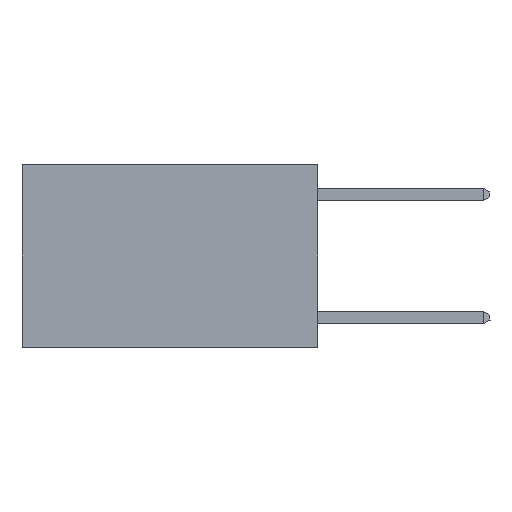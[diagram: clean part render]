
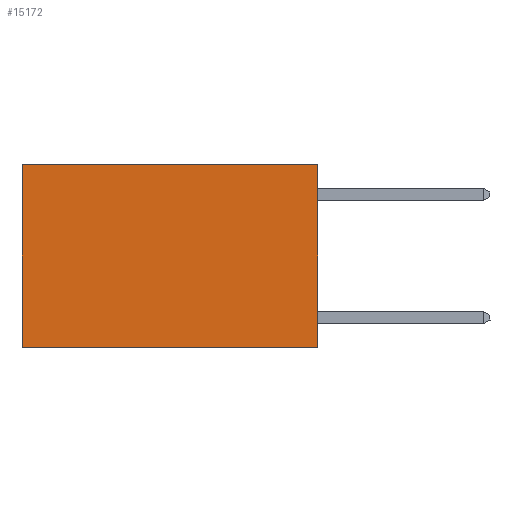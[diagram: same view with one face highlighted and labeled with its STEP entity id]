
A CAD part, left-side view. The second image highlights one B-rep face of the part: STEP entity #15172.
In plain terms, the highlighted planar face has unit normal (-1, 0, 0).
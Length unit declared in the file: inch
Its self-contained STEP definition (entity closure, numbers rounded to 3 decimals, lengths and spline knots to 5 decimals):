
#1443 = DIRECTION ( 'NONE',  ( 0., 1., 0. ) ) ;
#1890 = VECTOR ( 'NONE', #13519, 39.37008 ) ;
#2534 = AXIS2_PLACEMENT_3D ( 'NONE', #2882, #6406, #18572 ) ;
#2811 = PLANE ( 'NONE',  #2534 ) ;
#2882 = CARTESIAN_POINT ( 'NONE',  ( 0.2625, 0., 0. ) ) ;
#3169 = CARTESIAN_POINT ( 'NONE',  ( 0.2625, 0., 0. ) ) ;
#3248 = CARTESIAN_POINT ( 'NONE',  ( 0.2625, 0., 0. ) ) ;
#3826 = EDGE_CURVE ( 'NONE', #6300, #4791, #15140, .T. ) ;
#4094 = LINE ( 'NONE', #8619, #17411 ) ;
#4542 = VECTOR ( 'NONE', #1443, 39.37008 ) ;
#4791 = VERTEX_POINT ( 'NONE', #16194 ) ;
#5878 = VECTOR ( 'NONE', #15478, 39.37008 ) ;
#6300 = VERTEX_POINT ( 'NONE', #3169 ) ;
#6406 = DIRECTION ( 'NONE',  ( 1., 0., 0. ) ) ;
#8225 = CARTESIAN_POINT ( 'NONE',  ( 0.2625, 0., -0.37 ) ) ;
#8478 = VERTEX_POINT ( 'NONE', #9178 ) ;
#8619 = CARTESIAN_POINT ( 'NONE',  ( 0.2625, 0.6, 0. ) ) ;
#9178 = CARTESIAN_POINT ( 'NONE',  ( 0.2625, 0.6, -0.37 ) ) ;
#10360 = DIRECTION ( 'NONE',  ( 0., 0., -1. ) ) ;
#12296 = EDGE_CURVE ( 'NONE', #6300, #15762, #17868, .T. ) ;
#13203 = ORIENTED_EDGE ( 'NONE', *, *, #12296, .T. ) ;
#13519 = DIRECTION ( 'NONE',  ( 0., 1., 0. ) ) ;
#15140 = LINE ( 'NONE', #3248, #5878 ) ;
#15172 = ADVANCED_FACE ( 'NONE', ( #20125 ), #2811, .F. ) ;
#15426 = ORIENTED_EDGE ( 'NONE', *, *, #22498, .F. ) ;
#15478 = DIRECTION ( 'NONE',  ( 0., 0., -1. ) ) ;
#15762 = VERTEX_POINT ( 'NONE', #22079 ) ;
#15825 = LINE ( 'NONE', #8225, #1890 ) ;
#16194 = CARTESIAN_POINT ( 'NONE',  ( 0.2625, 0., -0.37 ) ) ;
#17237 = EDGE_CURVE ( 'NONE', #15762, #8478, #4094, .T. ) ;
#17411 = VECTOR ( 'NONE', #10360, 39.37008 ) ;
#17868 = LINE ( 'NONE', #22225, #4542 ) ;
#18301 = ORIENTED_EDGE ( 'NONE', *, *, #17237, .T. ) ;
#18572 = DIRECTION ( 'NONE',  ( 0., 0., -1. ) ) ;
#20125 = FACE_OUTER_BOUND ( 'NONE', #21129, .T. ) ;
#21106 = ORIENTED_EDGE ( 'NONE', *, *, #3826, .F. ) ;
#21129 = EDGE_LOOP ( 'NONE', ( #18301, #15426, #21106, #13203 ) ) ;
#22079 = CARTESIAN_POINT ( 'NONE',  ( 0.2625, 0.6, 0. ) ) ;
#22225 = CARTESIAN_POINT ( 'NONE',  ( 0.2625, 0., 0. ) ) ;
#22498 = EDGE_CURVE ( 'NONE', #4791, #8478, #15825, .T. ) ;
